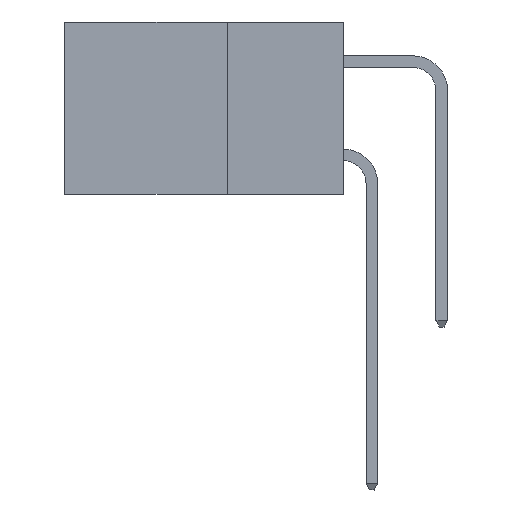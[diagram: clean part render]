
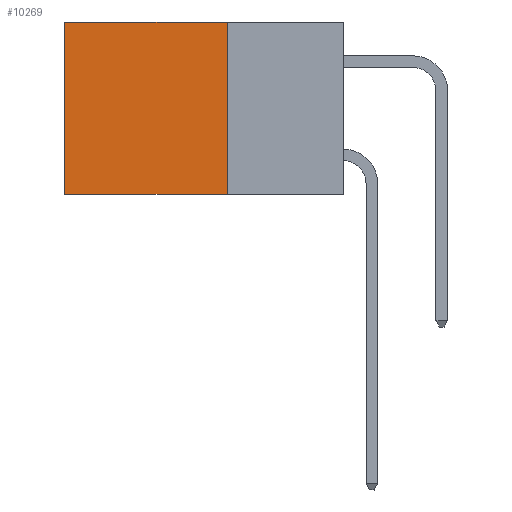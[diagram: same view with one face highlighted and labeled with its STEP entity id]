
A CAD part, left-side view. The second image highlights one B-rep face of the part: STEP entity #10269.
In plain terms, the highlighted planar face has unit normal (-1, 0, 0).
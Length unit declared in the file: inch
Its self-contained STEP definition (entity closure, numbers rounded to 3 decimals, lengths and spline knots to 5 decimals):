
#137 = VERTEX_POINT ( 'NONE', #20024 ) ;
#1602 = CARTESIAN_POINT ( 'NONE',  ( 0.298, 0.25, 0. ) ) ;
#1743 = DIRECTION ( 'NONE',  ( 0., 1., 0. ) ) ;
#2428 = ORIENTED_EDGE ( 'NONE', *, *, #6251, .T. ) ;
#2567 = VECTOR ( 'NONE', #10468, 39.37008 ) ;
#4798 = CARTESIAN_POINT ( 'NONE',  ( 0.298, 0.25, 0. ) ) ;
#5187 = LINE ( 'NONE', #11764, #13457 ) ;
#5350 = ORIENTED_EDGE ( 'NONE', *, *, #5884, .T. ) ;
#5487 = EDGE_CURVE ( 'NONE', #6087, #5500, #21266, .T. ) ;
#5500 = VERTEX_POINT ( 'NONE', #7742 ) ;
#5884 = EDGE_CURVE ( 'NONE', #7577, #137, #15761, .T. ) ;
#6087 = VERTEX_POINT ( 'NONE', #1602 ) ;
#6251 = EDGE_CURVE ( 'NONE', #6087, #7577, #5187, .T. ) ;
#6521 = AXIS2_PLACEMENT_3D ( 'NONE', #8401, #6823, #15091 ) ;
#6528 = VECTOR ( 'NONE', #7531, 39.37008 ) ;
#6823 = DIRECTION ( 'NONE',  ( 1., 0., 0. ) ) ;
#7531 = DIRECTION ( 'NONE',  ( 0., 0., -1. ) ) ;
#7577 = VERTEX_POINT ( 'NONE', #9068 ) ;
#7631 = DIRECTION ( 'NONE',  ( 0., 1., 0. ) ) ;
#7742 = CARTESIAN_POINT ( 'NONE',  ( 0.298, 0.25, -0.37 ) ) ;
#8401 = CARTESIAN_POINT ( 'NONE',  ( 0.298, 0.25, 0. ) ) ;
#9068 = CARTESIAN_POINT ( 'NONE',  ( 0.298, 0.6, 0. ) ) ;
#9105 = LINE ( 'NONE', #12488, #14006 ) ;
#10269 = ADVANCED_FACE ( 'NONE', ( #10463 ), #11821, .F. ) ;
#10463 = FACE_OUTER_BOUND ( 'NONE', #14782, .T. ) ;
#10468 = DIRECTION ( 'NONE',  ( 0., 0., -1. ) ) ;
#11764 = CARTESIAN_POINT ( 'NONE',  ( 0.298, 0.25, 0. ) ) ;
#11821 = PLANE ( 'NONE',  #6521 ) ;
#12488 = CARTESIAN_POINT ( 'NONE',  ( 0.298, 0.25, -0.37 ) ) ;
#13457 = VECTOR ( 'NONE', #1743, 39.37008 ) ;
#14006 = VECTOR ( 'NONE', #7631, 39.37008 ) ;
#14782 = EDGE_LOOP ( 'NONE', ( #5350, #16055, #18925, #2428 ) ) ;
#15091 = DIRECTION ( 'NONE',  ( 0., 0., -1. ) ) ;
#15761 = LINE ( 'NONE', #18837, #2567 ) ;
#16055 = ORIENTED_EDGE ( 'NONE', *, *, #19137, .F. ) ;
#18837 = CARTESIAN_POINT ( 'NONE',  ( 0.298, 0.6, 0. ) ) ;
#18925 = ORIENTED_EDGE ( 'NONE', *, *, #5487, .F. ) ;
#19137 = EDGE_CURVE ( 'NONE', #5500, #137, #9105, .T. ) ;
#20024 = CARTESIAN_POINT ( 'NONE',  ( 0.298, 0.6, -0.37 ) ) ;
#21266 = LINE ( 'NONE', #4798, #6528 ) ;
